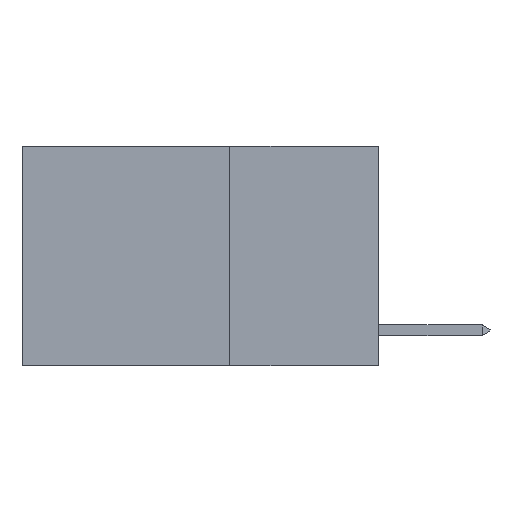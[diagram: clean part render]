
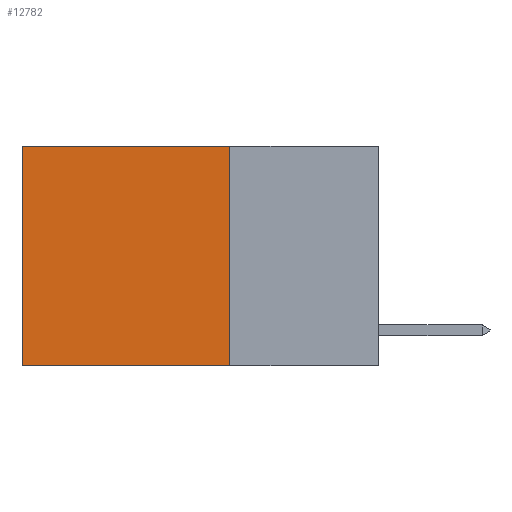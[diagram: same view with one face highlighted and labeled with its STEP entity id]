
A CAD part, left-side view. The second image highlights one B-rep face of the part: STEP entity #12782.
In plain terms, the highlighted planar face has unit normal (-1, 0, 0).
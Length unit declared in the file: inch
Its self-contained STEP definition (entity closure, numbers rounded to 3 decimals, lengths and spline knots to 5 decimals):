
#2120 = ORIENTED_EDGE ( 'NONE', *, *, #18939, .F. ) ;
#2523 = DIRECTION ( 'NONE',  ( 0., 0., -1. ) ) ;
#3179 = VECTOR ( 'NONE', #2523, 39.37008 ) ;
#4803 = ORIENTED_EDGE ( 'NONE', *, *, #19745, .T. ) ;
#5160 = VECTOR ( 'NONE', #24015, 39.37008 ) ;
#5298 = DIRECTION ( 'NONE',  ( 0., 0., -1. ) ) ;
#5842 = VERTEX_POINT ( 'NONE', #18333 ) ;
#8968 = DIRECTION ( 'NONE',  ( 0., 1., 0. ) ) ;
#9283 = LINE ( 'NONE', #13088, #25351 ) ;
#10417 = CARTESIAN_POINT ( 'NONE',  ( 0.2625, 0.25, 0. ) ) ;
#10793 = VERTEX_POINT ( 'NONE', #10417 ) ;
#10868 = LINE ( 'NONE', #19808, #5160 ) ;
#12782 = ADVANCED_FACE ( 'NONE', ( #25082 ), #26317, .F. ) ;
#13088 = CARTESIAN_POINT ( 'NONE',  ( 0.2625, 0.25, -0.37 ) ) ;
#14496 = EDGE_CURVE ( 'NONE', #10793, #5842, #20056, .T. ) ;
#15187 = DIRECTION ( 'NONE',  ( 0., 1., 0. ) ) ;
#17443 = CARTESIAN_POINT ( 'NONE',  ( 0.2625, 0.25, 0. ) ) ;
#17980 = DIRECTION ( 'NONE',  ( 1., 0., 0. ) ) ;
#18034 = CARTESIAN_POINT ( 'NONE',  ( 0.2625, 0.6, 0. ) ) ;
#18333 = CARTESIAN_POINT ( 'NONE',  ( 0.2625, 0.25, -0.37 ) ) ;
#18400 = VECTOR ( 'NONE', #8968, 39.37008 ) ;
#18939 = EDGE_CURVE ( 'NONE', #5842, #26076, #9283, .T. ) ;
#19631 = EDGE_CURVE ( 'NONE', #10793, #24478, #23984, .T. ) ;
#19745 = EDGE_CURVE ( 'NONE', #24478, #26076, #10868, .T. ) ;
#19808 = CARTESIAN_POINT ( 'NONE',  ( 0.2625, 0.6, 0. ) ) ;
#20056 = LINE ( 'NONE', #17443, #3179 ) ;
#20775 = EDGE_LOOP ( 'NONE', ( #4803, #2120, #26971, #26280 ) ) ;
#22210 = AXIS2_PLACEMENT_3D ( 'NONE', #26227, #17980, #5298 ) ;
#23635 = CARTESIAN_POINT ( 'NONE',  ( 0.2625, 0.6, -0.37 ) ) ;
#23652 = CARTESIAN_POINT ( 'NONE',  ( 0.2625, 0.25, 0. ) ) ;
#23984 = LINE ( 'NONE', #23652, #18400 ) ;
#24015 = DIRECTION ( 'NONE',  ( 0., 0., -1. ) ) ;
#24478 = VERTEX_POINT ( 'NONE', #18034 ) ;
#25082 = FACE_OUTER_BOUND ( 'NONE', #20775, .T. ) ;
#25351 = VECTOR ( 'NONE', #15187, 39.37008 ) ;
#26076 = VERTEX_POINT ( 'NONE', #23635 ) ;
#26227 = CARTESIAN_POINT ( 'NONE',  ( 0.2625, 0.25, 0. ) ) ;
#26280 = ORIENTED_EDGE ( 'NONE', *, *, #19631, .T. ) ;
#26317 = PLANE ( 'NONE',  #22210 ) ;
#26971 = ORIENTED_EDGE ( 'NONE', *, *, #14496, .F. ) ;
